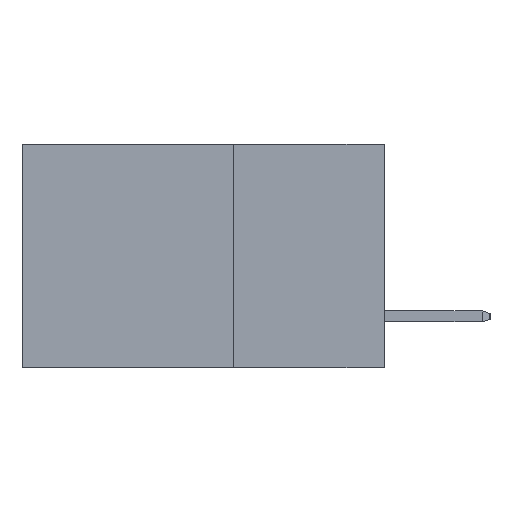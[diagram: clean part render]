
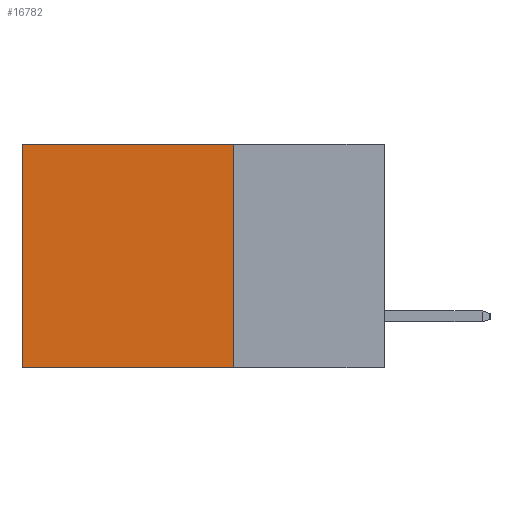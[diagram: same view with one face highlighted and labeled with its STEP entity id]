
A CAD part, left-side view. The second image highlights one B-rep face of the part: STEP entity #16782.
In plain terms, the highlighted planar face has unit normal (-1, 0, 0).
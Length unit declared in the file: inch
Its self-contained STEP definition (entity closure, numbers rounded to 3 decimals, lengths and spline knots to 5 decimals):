
#910 = CARTESIAN_POINT ( 'NONE',  ( 0.298, 0.6, -0.37 ) ) ;
#1041 = VERTEX_POINT ( 'NONE', #910 ) ;
#1151 = FACE_OUTER_BOUND ( 'NONE', #9120, .T. ) ;
#1650 = CARTESIAN_POINT ( 'NONE',  ( 0.298, 0.25, 0. ) ) ;
#2373 = ORIENTED_EDGE ( 'NONE', *, *, #17699, .F. ) ;
#2437 = VERTEX_POINT ( 'NONE', #1650 ) ;
#3248 = LINE ( 'NONE', #18309, #16703 ) ;
#3946 = AXIS2_PLACEMENT_3D ( 'NONE', #6265, #4513, #16792 ) ;
#4513 = DIRECTION ( 'NONE',  ( 1., 0., 0. ) ) ;
#4542 = VECTOR ( 'NONE', #20676, 39.37008 ) ;
#5416 = CARTESIAN_POINT ( 'NONE',  ( 0.298, 0.25, -0.37 ) ) ;
#6265 = CARTESIAN_POINT ( 'NONE',  ( 0.298, 0.25, 0. ) ) ;
#6916 = LINE ( 'NONE', #10299, #16225 ) ;
#7178 = DIRECTION ( 'NONE',  ( 0., 1., 0. ) ) ;
#8081 = ORIENTED_EDGE ( 'NONE', *, *, #22662, .T. ) ;
#9120 = EDGE_LOOP ( 'NONE', ( #8081, #17653, #2373, #11535 ) ) ;
#9621 = DIRECTION ( 'NONE',  ( 0., 1., 0. ) ) ;
#10253 = CARTESIAN_POINT ( 'NONE',  ( 0.298, 0.6, 0. ) ) ;
#10299 = CARTESIAN_POINT ( 'NONE',  ( 0.298, 0.6, 0. ) ) ;
#10543 = VECTOR ( 'NONE', #7178, 39.37008 ) ;
#11535 = ORIENTED_EDGE ( 'NONE', *, *, #13286, .T. ) ;
#13286 = EDGE_CURVE ( 'NONE', #2437, #17691, #19259, .T. ) ;
#13786 = CARTESIAN_POINT ( 'NONE',  ( 0.298, 0.25, 0. ) ) ;
#14106 = LINE ( 'NONE', #13786, #4542 ) ;
#14121 = CARTESIAN_POINT ( 'NONE',  ( 0.298, 0.25, 0. ) ) ;
#14873 = EDGE_CURVE ( 'NONE', #19649, #1041, #3248, .T. ) ;
#15046 = PLANE ( 'NONE',  #3946 ) ;
#16225 = VECTOR ( 'NONE', #22434, 39.37008 ) ;
#16703 = VECTOR ( 'NONE', #9621, 39.37008 ) ;
#16782 = ADVANCED_FACE ( 'NONE', ( #1151 ), #15046, .F. ) ;
#16792 = DIRECTION ( 'NONE',  ( 0., 0., -1. ) ) ;
#17653 = ORIENTED_EDGE ( 'NONE', *, *, #14873, .F. ) ;
#17691 = VERTEX_POINT ( 'NONE', #10253 ) ;
#17699 = EDGE_CURVE ( 'NONE', #2437, #19649, #14106, .T. ) ;
#18309 = CARTESIAN_POINT ( 'NONE',  ( 0.298, 0.25, -0.37 ) ) ;
#19259 = LINE ( 'NONE', #14121, #10543 ) ;
#19649 = VERTEX_POINT ( 'NONE', #5416 ) ;
#20676 = DIRECTION ( 'NONE',  ( 0., 0., -1. ) ) ;
#22434 = DIRECTION ( 'NONE',  ( 0., 0., -1. ) ) ;
#22662 = EDGE_CURVE ( 'NONE', #17691, #1041, #6916, .T. ) ;
